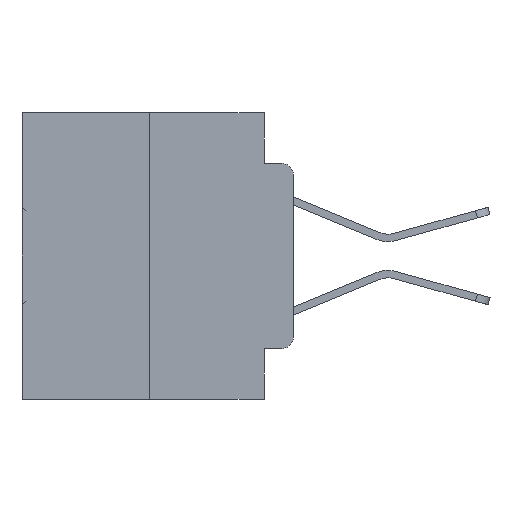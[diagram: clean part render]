
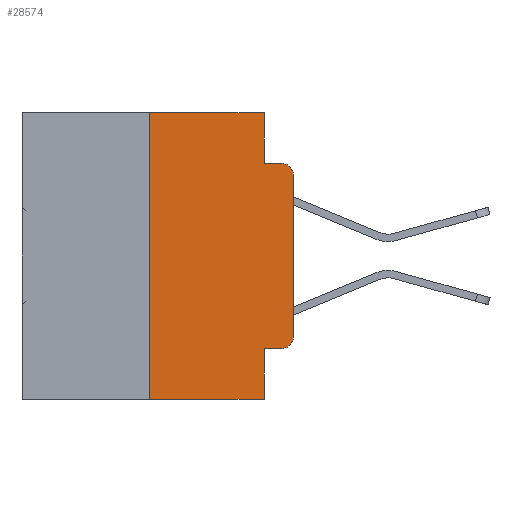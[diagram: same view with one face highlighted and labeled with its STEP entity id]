
A CAD part, left-side view. The second image highlights one B-rep face of the part: STEP entity #28574.
In plain terms, the highlighted planar face has unit normal (-1, 0, 0).
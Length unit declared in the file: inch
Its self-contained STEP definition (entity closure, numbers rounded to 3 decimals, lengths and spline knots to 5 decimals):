
#37 = CARTESIAN_POINT ( 'NONE',  ( 0., 0.051, -0.5 ) ) ;
#126 = ORIENTED_EDGE ( 'NONE', *, *, #30005, .T. ) ;
#2094 = CARTESIAN_POINT ( 'NONE',  ( 0., 0., -0.1085 ) ) ;
#2286 = DIRECTION ( 'NONE',  ( 1., 0., 0. ) ) ;
#2718 = ORIENTED_EDGE ( 'NONE', *, *, #2779, .T. ) ;
#2779 = EDGE_CURVE ( 'NONE', #12408, #12050, #15029, .T. ) ;
#3570 = ORIENTED_EDGE ( 'NONE', *, *, #4753, .F. ) ;
#4429 = CARTESIAN_POINT ( 'NONE',  ( 0., 0.02, -0.1085 ) ) ;
#4672 = EDGE_CURVE ( 'NONE', #32479, #33066, #17372, .T. ) ;
#4753 = EDGE_CURVE ( 'NONE', #25736, #19638, #8454, .T. ) ;
#4766 = DIRECTION ( 'NONE',  ( 0., 0., -1. ) ) ;
#5335 = CARTESIAN_POINT ( 'NONE',  ( 0., 0.02, -0.3915 ) ) ;
#5752 = DIRECTION ( 'NONE',  ( -1., 0., 0. ) ) ;
#5793 = CARTESIAN_POINT ( 'NONE',  ( 0., 0.051, -0.4115 ) ) ;
#6276 = CARTESIAN_POINT ( 'NONE',  ( 0., 0.02, -0.4115 ) ) ;
#6374 = AXIS2_PLACEMENT_3D ( 'NONE', #5335, #5752, #28932 ) ;
#6478 = LINE ( 'NONE', #24441, #33025 ) ;
#6723 = CARTESIAN_POINT ( 'NONE',  ( 0., 0.25, 0. ) ) ;
#7672 = VECTOR ( 'NONE', #23934, 39.37008 ) ;
#7914 = DIRECTION ( 'NONE',  ( 0., -1., 0. ) ) ;
#8161 = LINE ( 'NONE', #18254, #26706 ) ;
#8454 = LINE ( 'NONE', #21454, #7672 ) ;
#10486 = VECTOR ( 'NONE', #31031, 39.37008 ) ;
#11231 = LINE ( 'NONE', #23493, #16876 ) ;
#11386 = AXIS2_PLACEMENT_3D ( 'NONE', #4429, #11950, #29922 ) ;
#11950 = DIRECTION ( 'NONE',  ( -1., 0., 0. ) ) ;
#12050 = VERTEX_POINT ( 'NONE', #2094 ) ;
#12077 = CARTESIAN_POINT ( 'NONE',  ( 0., 0., 0. ) ) ;
#12408 = VERTEX_POINT ( 'NONE', #26765 ) ;
#12618 = VERTEX_POINT ( 'NONE', #6276 ) ;
#12655 = CIRCLE ( 'NONE', #6374, 0.02 ) ;
#12768 = ORIENTED_EDGE ( 'NONE', *, *, #14744, .F. ) ;
#13599 = EDGE_CURVE ( 'NONE', #12050, #33066, #28553, .T. ) ;
#13700 = ORIENTED_EDGE ( 'NONE', *, *, #13599, .T. ) ;
#13874 = DIRECTION ( 'NONE',  ( 0., 0., -1. ) ) ;
#14744 = EDGE_CURVE ( 'NONE', #18746, #26231, #11231, .T. ) ;
#15029 = LINE ( 'NONE', #12077, #23818 ) ;
#15584 = LINE ( 'NONE', #15887, #19180 ) ;
#15623 = EDGE_CURVE ( 'NONE', #30426, #18746, #15584, .T. ) ;
#15826 = LINE ( 'NONE', #24081, #17099 ) ;
#15887 = CARTESIAN_POINT ( 'NONE',  ( 0., 0.25, 0. ) ) ;
#16302 = AXIS2_PLACEMENT_3D ( 'NONE', #30591, #2286, #4766 ) ;
#16876 = VECTOR ( 'NONE', #23727, 39.37008 ) ;
#17099 = VECTOR ( 'NONE', #13874, 39.37008 ) ;
#17372 = LINE ( 'NONE', #28472, #10486 ) ;
#18254 = CARTESIAN_POINT ( 'NONE',  ( 0., 0.051, -0.4115 ) ) ;
#18746 = VERTEX_POINT ( 'NONE', #6723 ) ;
#19180 = VECTOR ( 'NONE', #23495, 39.37008 ) ;
#19638 = VERTEX_POINT ( 'NONE', #37 ) ;
#19696 = ORIENTED_EDGE ( 'NONE', *, *, #31443, .T. ) ;
#19824 = CARTESIAN_POINT ( 'NONE',  ( 0., 0.25, -0.5 ) ) ;
#20084 = ORIENTED_EDGE ( 'NONE', *, *, #30101, .F. ) ;
#20142 = DIRECTION ( 'NONE',  ( 0., 0., 1. ) ) ;
#21454 = CARTESIAN_POINT ( 'NONE',  ( 0., 0.051, 0. ) ) ;
#23207 = ORIENTED_EDGE ( 'NONE', *, *, #23526, .T. ) ;
#23493 = CARTESIAN_POINT ( 'NONE',  ( 0., 0.473, 0. ) ) ;
#23495 = DIRECTION ( 'NONE',  ( 0., 0., 1. ) ) ;
#23526 = EDGE_CURVE ( 'NONE', #25736, #12618, #8161, .T. ) ;
#23727 = DIRECTION ( 'NONE',  ( 0., -1., 0. ) ) ;
#23818 = VECTOR ( 'NONE', #20142, 39.37008 ) ;
#23934 = DIRECTION ( 'NONE',  ( 0., 0., -1. ) ) ;
#24081 = CARTESIAN_POINT ( 'NONE',  ( 0., 0.051, 0. ) ) ;
#24441 = CARTESIAN_POINT ( 'NONE',  ( 0., 0.473, -0.5 ) ) ;
#25736 = VERTEX_POINT ( 'NONE', #5793 ) ;
#25889 = CARTESIAN_POINT ( 'NONE',  ( 0., 0.051, 0. ) ) ;
#26061 = CARTESIAN_POINT ( 'NONE',  ( 0., 0.051, -0.0885 ) ) ;
#26231 = VERTEX_POINT ( 'NONE', #25889 ) ;
#26400 = FACE_OUTER_BOUND ( 'NONE', #33148, .T. ) ;
#26442 = ORIENTED_EDGE ( 'NONE', *, *, #4672, .F. ) ;
#26706 = VECTOR ( 'NONE', #7914, 39.37008 ) ;
#26765 = CARTESIAN_POINT ( 'NONE',  ( 0., 0., -0.3915 ) ) ;
#28420 = CARTESIAN_POINT ( 'NONE',  ( 0., 0.02, -0.0885 ) ) ;
#28472 = CARTESIAN_POINT ( 'NONE',  ( 0., 0.051, -0.0885 ) ) ;
#28553 = CIRCLE ( 'NONE', #11386, 0.02 ) ;
#28574 = ADVANCED_FACE ( 'NONE', ( #26400 ), #30474, .F. ) ;
#28619 = ORIENTED_EDGE ( 'NONE', *, *, #15623, .F. ) ;
#28932 = DIRECTION ( 'NONE',  ( 0., 0., -1. ) ) ;
#29922 = DIRECTION ( 'NONE',  ( 0., 0., -1. ) ) ;
#30005 = EDGE_CURVE ( 'NONE', #12618, #12408, #12655, .T. ) ;
#30101 = EDGE_CURVE ( 'NONE', #26231, #32479, #15826, .T. ) ;
#30426 = VERTEX_POINT ( 'NONE', #19824 ) ;
#30474 = PLANE ( 'NONE',  #16302 ) ;
#30591 = CARTESIAN_POINT ( 'NONE',  ( 0., 0.473, 0. ) ) ;
#31031 = DIRECTION ( 'NONE',  ( 0., -1., 0. ) ) ;
#31443 = EDGE_CURVE ( 'NONE', #30426, #19638, #6478, .T. ) ;
#32309 = DIRECTION ( 'NONE',  ( 0., -1., 0. ) ) ;
#32479 = VERTEX_POINT ( 'NONE', #26061 ) ;
#33025 = VECTOR ( 'NONE', #32309, 39.37008 ) ;
#33066 = VERTEX_POINT ( 'NONE', #28420 ) ;
#33148 = EDGE_LOOP ( 'NONE', ( #2718, #13700, #26442, #20084, #12768, #28619, #19696, #3570, #23207, #126 ) ) ;
